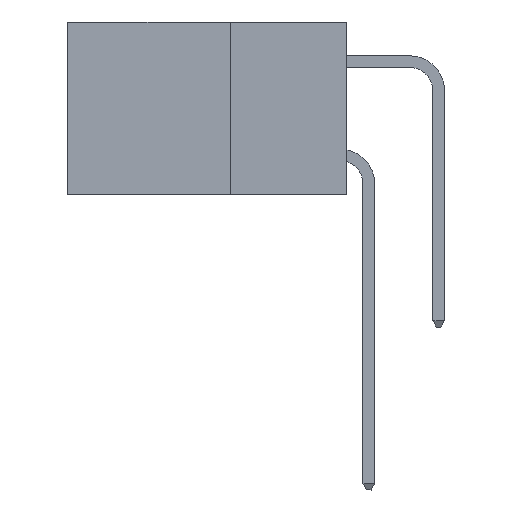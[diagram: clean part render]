
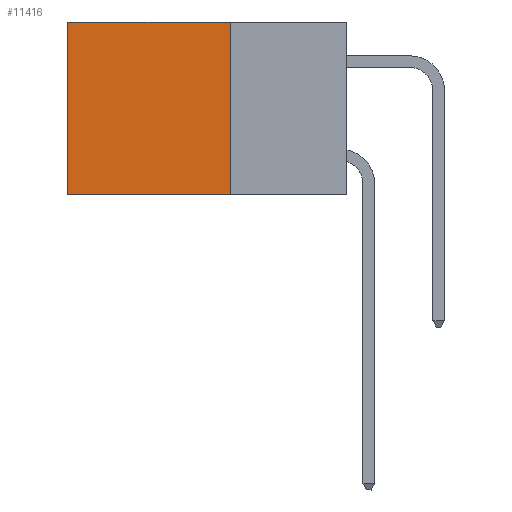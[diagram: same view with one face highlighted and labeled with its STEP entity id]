
A CAD part, left-side view. The second image highlights one B-rep face of the part: STEP entity #11416.
In plain terms, the highlighted planar face has unit normal (-1, 0, 0).
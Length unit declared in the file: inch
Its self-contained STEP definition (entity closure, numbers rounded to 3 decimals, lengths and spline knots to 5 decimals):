
#684 = DIRECTION ( 'NONE',  ( 0., 1., 0. ) ) ;
#782 = VECTOR ( 'NONE', #684, 39.37008 ) ;
#1132 = DIRECTION ( 'NONE',  ( 0., 1., 0. ) ) ;
#1653 = CARTESIAN_POINT ( 'NONE',  ( 0.2875, 0.25, 0. ) ) ;
#2068 = LINE ( 'NONE', #10097, #12845 ) ;
#2643 = EDGE_LOOP ( 'NONE', ( #12101, #6115, #4783, #13772 ) ) ;
#4108 = CARTESIAN_POINT ( 'NONE',  ( 0.2875, 0.6, 0. ) ) ;
#4783 = ORIENTED_EDGE ( 'NONE', *, *, #9193, .F. ) ;
#4819 = VERTEX_POINT ( 'NONE', #4108 ) ;
#4850 = CARTESIAN_POINT ( 'NONE',  ( 0.2875, 0.6, 0. ) ) ;
#4853 = VECTOR ( 'NONE', #1132, 39.37008 ) ;
#4923 = LINE ( 'NONE', #4850, #11635 ) ;
#5287 = VERTEX_POINT ( 'NONE', #7684 ) ;
#5314 = PLANE ( 'NONE',  #5561 ) ;
#5561 = AXIS2_PLACEMENT_3D ( 'NONE', #1653, #6409, #8936 ) ;
#6115 = ORIENTED_EDGE ( 'NONE', *, *, #13852, .F. ) ;
#6409 = DIRECTION ( 'NONE',  ( 1., 0., 0. ) ) ;
#6454 = CARTESIAN_POINT ( 'NONE',  ( 0.2875, 0.25, -0.37 ) ) ;
#7684 = CARTESIAN_POINT ( 'NONE',  ( 0.2875, 0.25, 0. ) ) ;
#7758 = CARTESIAN_POINT ( 'NONE',  ( 0.2875, 0.6, -0.37 ) ) ;
#8139 = LINE ( 'NONE', #10755, #782 ) ;
#8319 = DIRECTION ( 'NONE',  ( 0., 0., -1. ) ) ;
#8354 = VERTEX_POINT ( 'NONE', #7758 ) ;
#8467 = EDGE_CURVE ( 'NONE', #5287, #4819, #8139, .T. ) ;
#8936 = DIRECTION ( 'NONE',  ( 0., 0., -1. ) ) ;
#9193 = EDGE_CURVE ( 'NONE', #5287, #13491, #2068, .T. ) ;
#10097 = CARTESIAN_POINT ( 'NONE',  ( 0.2875, 0.25, 0. ) ) ;
#10704 = CARTESIAN_POINT ( 'NONE',  ( 0.2875, 0.25, -0.37 ) ) ;
#10755 = CARTESIAN_POINT ( 'NONE',  ( 0.2875, 0.25, 0. ) ) ;
#11287 = EDGE_CURVE ( 'NONE', #4819, #8354, #4923, .T. ) ;
#11416 = ADVANCED_FACE ( 'NONE', ( #12498 ), #5314, .F. ) ;
#11635 = VECTOR ( 'NONE', #12026, 39.37008 ) ;
#11908 = LINE ( 'NONE', #10704, #4853 ) ;
#12026 = DIRECTION ( 'NONE',  ( 0., 0., -1. ) ) ;
#12101 = ORIENTED_EDGE ( 'NONE', *, *, #11287, .T. ) ;
#12498 = FACE_OUTER_BOUND ( 'NONE', #2643, .T. ) ;
#12845 = VECTOR ( 'NONE', #8319, 39.37008 ) ;
#13491 = VERTEX_POINT ( 'NONE', #6454 ) ;
#13772 = ORIENTED_EDGE ( 'NONE', *, *, #8467, .T. ) ;
#13852 = EDGE_CURVE ( 'NONE', #13491, #8354, #11908, .T. ) ;
